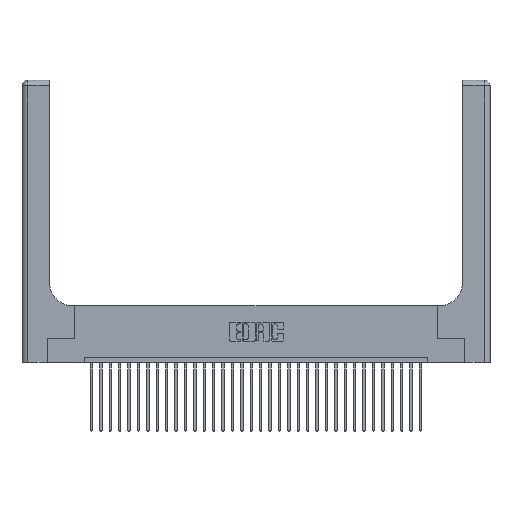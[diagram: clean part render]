
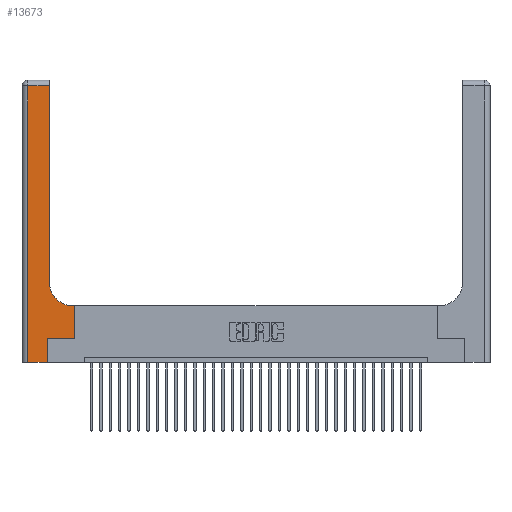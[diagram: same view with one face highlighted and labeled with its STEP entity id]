
A CAD part, top view. The second image highlights one B-rep face of the part: STEP entity #13673.
In plain terms, the highlighted planar face has unit normal (0, 0, 1).
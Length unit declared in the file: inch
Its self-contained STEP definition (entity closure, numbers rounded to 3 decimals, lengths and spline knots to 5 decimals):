
#61 = LINE ( 'NONE', #31954, #2101 ) ;
#849 = ORIENTED_EDGE ( 'NONE', *, *, #3026, .T. ) ;
#1058 = CARTESIAN_POINT ( 'NONE',  ( 0.2915, 3., 0.37 ) ) ;
#1163 = VERTEX_POINT ( 'NONE', #2055 ) ;
#1176 = DIRECTION ( 'NONE',  ( -1., 0., 0. ) ) ;
#1309 = DIRECTION ( 'NONE',  ( 0., 1., 0. ) ) ;
#1352 = DIRECTION ( 'NONE',  ( 1., 0., 0. ) ) ;
#1429 = ORIENTED_EDGE ( 'NONE', *, *, #15558, .T. ) ;
#1447 = CARTESIAN_POINT ( 'NONE',  ( 0.269, 0.25, 0.37 ) ) ;
#1853 = CARTESIAN_POINT ( 'NONE',  ( 0.269, 0.25, 0.37 ) ) ;
#2055 = CARTESIAN_POINT ( 'NONE',  ( 0.06, 0., 0.37 ) ) ;
#2101 = VECTOR ( 'NONE', #1352, 39.37008 ) ;
#2934 = EDGE_CURVE ( 'NONE', #1163, #29156, #61, .T. ) ;
#3026 = EDGE_CURVE ( 'NONE', #31706, #10231, #4839, .T. ) ;
#3974 = CARTESIAN_POINT ( 'NONE',  ( 0.06, 2.94, 0.37 ) ) ;
#4731 = ORIENTED_EDGE ( 'NONE', *, *, #7883, .T. ) ;
#4839 = LINE ( 'NONE', #10746, #14881 ) ;
#5294 = VECTOR ( 'NONE', #1309, 39.37008 ) ;
#5667 = CARTESIAN_POINT ( 'NONE',  ( 0.5415, 0.6, 0.37 ) ) ;
#6232 = LINE ( 'NONE', #1447, #10226 ) ;
#7883 = EDGE_CURVE ( 'NONE', #29156, #18580, #17900, .T. ) ;
#9149 = CARTESIAN_POINT ( 'NONE',  ( 0.2915, 0.85, 0.37 ) ) ;
#9592 = ORIENTED_EDGE ( 'NONE', *, *, #29381, .T. ) ;
#9676 = DIRECTION ( 'NONE',  ( 0., -1., 0. ) ) ;
#10192 = CIRCLE ( 'NONE', #19626, 0.25 ) ;
#10226 = VECTOR ( 'NONE', #19271, 39.37008 ) ;
#10231 = VERTEX_POINT ( 'NONE', #5667 ) ;
#10746 = CARTESIAN_POINT ( 'NONE',  ( 0.2915, 0.6, 0.37 ) ) ;
#10864 = DIRECTION ( 'NONE',  ( -1., 0., 0. ) ) ;
#11125 = CARTESIAN_POINT ( 'NONE',  ( 0.269, 0., 0.37 ) ) ;
#12181 = LINE ( 'NONE', #20540, #14602 ) ;
#13673 = ADVANCED_FACE ( 'NONE', ( #14006 ), #26797, .F. ) ;
#13911 = LINE ( 'NONE', #32401, #26646 ) ;
#14006 = FACE_OUTER_BOUND ( 'NONE', #15521, .T. ) ;
#14602 = VECTOR ( 'NONE', #25662, 39.37008 ) ;
#14881 = VECTOR ( 'NONE', #10864, 39.37008 ) ;
#15521 = EDGE_LOOP ( 'NONE', ( #21793, #22426, #1429, #32254, #4731, #9592, #19486, #849, #19327 ) ) ;
#15558 = EDGE_CURVE ( 'NONE', #26832, #1163, #13911, .T. ) ;
#16344 = DIRECTION ( 'NONE',  ( 1., 0., 0. ) ) ;
#17240 = VERTEX_POINT ( 'NONE', #24888 ) ;
#17317 = LINE ( 'NONE', #31669, #5294 ) ;
#17900 = LINE ( 'NONE', #19447, #26661 ) ;
#18580 = VERTEX_POINT ( 'NONE', #1853 ) ;
#19271 = DIRECTION ( 'NONE',  ( 1., 0., 0. ) ) ;
#19327 = ORIENTED_EDGE ( 'NONE', *, *, #29843, .T. ) ;
#19447 = CARTESIAN_POINT ( 'NONE',  ( 0.269, 0., 0.37 ) ) ;
#19486 = ORIENTED_EDGE ( 'NONE', *, *, #31100, .T. ) ;
#19626 = AXIS2_PLACEMENT_3D ( 'NONE', #29294, #26593, #16344 ) ;
#20129 = VERTEX_POINT ( 'NONE', #21639 ) ;
#20540 = CARTESIAN_POINT ( 'NONE',  ( 0., 2.94, 0.37 ) ) ;
#21639 = CARTESIAN_POINT ( 'NONE',  ( 0.2915, 2.94, 0.37 ) ) ;
#21765 = CARTESIAN_POINT ( 'NONE',  ( 0., 3., 0.37 ) ) ;
#21793 = ORIENTED_EDGE ( 'NONE', *, *, #28475, .T. ) ;
#21897 = DIRECTION ( 'NONE',  ( 0., 1., 0. ) ) ;
#22426 = ORIENTED_EDGE ( 'NONE', *, *, #23938, .T. ) ;
#23938 = EDGE_CURVE ( 'NONE', #20129, #26832, #12181, .T. ) ;
#24103 = DIRECTION ( 'NONE',  ( 0., 1., 0. ) ) ;
#24314 = CARTESIAN_POINT ( 'NONE',  ( 0.5585, 0.6, 0.37 ) ) ;
#24888 = CARTESIAN_POINT ( 'NONE',  ( 0.5585, 0.25, 0.37 ) ) ;
#25662 = DIRECTION ( 'NONE',  ( -1., 0., 0. ) ) ;
#26593 = DIRECTION ( 'NONE',  ( 0., 0., -1. ) ) ;
#26646 = VECTOR ( 'NONE', #9676, 39.37008 ) ;
#26661 = VECTOR ( 'NONE', #21897, 39.37008 ) ;
#26797 = PLANE ( 'NONE',  #31332 ) ;
#26832 = VERTEX_POINT ( 'NONE', #3974 ) ;
#28475 = EDGE_CURVE ( 'NONE', #28652, #20129, #31092, .T. ) ;
#28652 = VERTEX_POINT ( 'NONE', #9149 ) ;
#29156 = VERTEX_POINT ( 'NONE', #11125 ) ;
#29294 = CARTESIAN_POINT ( 'NONE',  ( 0.5415, 0.85, 0.37 ) ) ;
#29381 = EDGE_CURVE ( 'NONE', #18580, #17240, #6232, .T. ) ;
#29843 = EDGE_CURVE ( 'NONE', #10231, #28652, #10192, .T. ) ;
#31092 = LINE ( 'NONE', #1058, #31485 ) ;
#31100 = EDGE_CURVE ( 'NONE', #17240, #31706, #17317, .T. ) ;
#31332 = AXIS2_PLACEMENT_3D ( 'NONE', #21765, #31748, #1176 ) ;
#31485 = VECTOR ( 'NONE', #24103, 39.37008 ) ;
#31669 = CARTESIAN_POINT ( 'NONE',  ( 0.5585, 0.25, 0.37 ) ) ;
#31706 = VERTEX_POINT ( 'NONE', #24314 ) ;
#31748 = DIRECTION ( 'NONE',  ( 0., 0., -1. ) ) ;
#31954 = CARTESIAN_POINT ( 'NONE',  ( 0., 0., 0.37 ) ) ;
#32254 = ORIENTED_EDGE ( 'NONE', *, *, #2934, .T. ) ;
#32401 = CARTESIAN_POINT ( 'NONE',  ( 0.06, 3., 0.37 ) ) ;
